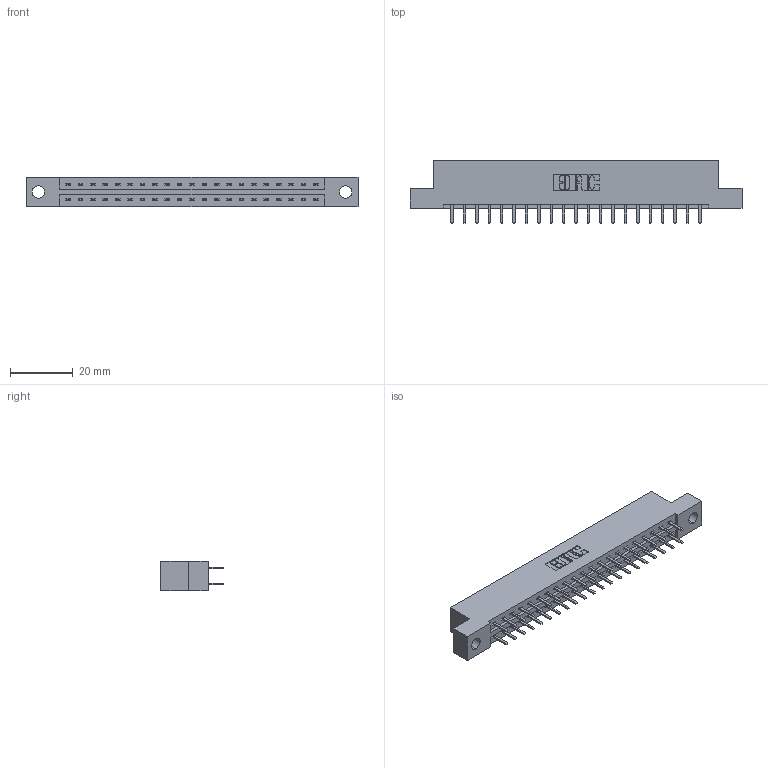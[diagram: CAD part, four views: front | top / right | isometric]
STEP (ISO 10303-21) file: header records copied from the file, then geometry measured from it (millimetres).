
FILE_DESCRIPTION (( 'STEP AP203' ), '1' );
FILE_NAME ('337-042-520-204.STEP', '2019-10-09T12:01:06', ( '' ), ( '' ), 'SwSTEP 2.0', 'SolidWorks 2016', '' );
FILE_SCHEMA (( 'CONFIG_CONTROL_DESIGN' ));
Length unit declared in the file: inch
Products named in the file (3): 337-042-520-204; 337 Part_Flush Mounting Lugs - 0.156 Dia-TH; 345-292-001_345-293-120
Assembly tree (43 placements, depth 2):
  337-042-520-204
    337 Part_Flush Mounting Lugs - 0.156 Dia-TH
    345-292-001_345-293-120  x42
Bounding box: 106.22 x 20.02 x 9.4 mm (x, y, z)
Volume: 10808.7 mm3; surface area: 11760.1 mm2
Topology: 43 solids, 43 shells, 2550 faces, 7409 edges, 4826 vertices
Faces by surface type: plane 1750, cylinder 800
Entity records: 19115 total; most frequent: CARTESIAN_POINT 3250, ORIENTED_EDGE 3174, DIRECTION 2791, EDGE_CURVE 1587, VECTOR 1455, LINE 1455, VERTEX_POINT 1054, AXIS2_PLACEMENT_3D 668
